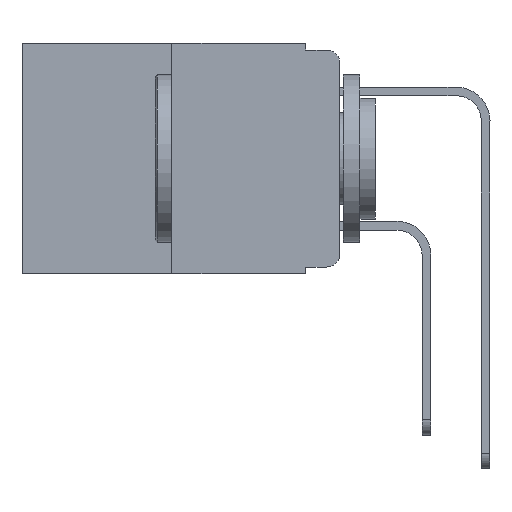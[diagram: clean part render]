
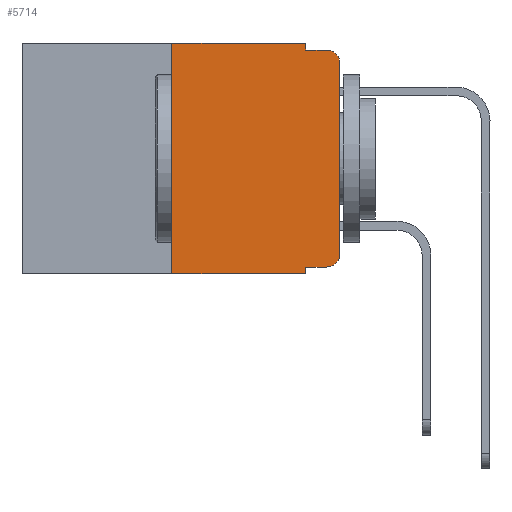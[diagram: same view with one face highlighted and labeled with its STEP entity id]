
A CAD part, left-side view. The second image highlights one B-rep face of the part: STEP entity #5714.
In plain terms, the highlighted planar face has unit normal (-1, 0, 0).
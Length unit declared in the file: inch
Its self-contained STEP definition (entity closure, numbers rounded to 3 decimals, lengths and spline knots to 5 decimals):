
#131 = VERTEX_POINT ( 'NONE', #2396 ) ;
#671 = CARTESIAN_POINT ( 'NONE',  ( 0., 0.051, 0. ) ) ;
#783 = AXIS2_PLACEMENT_3D ( 'NONE', #6863, #4051, #10195 ) ;
#1000 = DIRECTION ( 'NONE',  ( 0., 0., -1. ) ) ;
#1332 = LINE ( 'NONE', #9382, #6389 ) ;
#1361 = LINE ( 'NONE', #9855, #4149 ) ;
#1840 = CARTESIAN_POINT ( 'NONE',  ( 0., 0.25, 0. ) ) ;
#2251 = VERTEX_POINT ( 'NONE', #11145 ) ;
#2294 = DIRECTION ( 'NONE',  ( 0., -1., 0. ) ) ;
#2305 = EDGE_CURVE ( 'NONE', #131, #3315, #7604, .T. ) ;
#2396 = CARTESIAN_POINT ( 'NONE',  ( 0., 0.25, 0. ) ) ;
#2645 = CARTESIAN_POINT ( 'NONE',  ( 0., 0.051, 0. ) ) ;
#2754 = VECTOR ( 'NONE', #7580, 39.37008 ) ;
#2780 = ORIENTED_EDGE ( 'NONE', *, *, #8058, .T. ) ;
#2815 = ORIENTED_EDGE ( 'NONE', *, *, #8389, .T. ) ;
#2819 = EDGE_CURVE ( 'NONE', #5013, #5058, #1361, .T. ) ;
#2856 = ORIENTED_EDGE ( 'NONE', *, *, #8532, .F. ) ;
#2894 = ORIENTED_EDGE ( 'NONE', *, *, #8659, .F. ) ;
#2931 = ORIENTED_EDGE ( 'NONE', *, *, #2305, .F. ) ;
#3083 = PLANE ( 'NONE',  #783 ) ;
#3235 = ORIENTED_EDGE ( 'NONE', *, *, #8673, .F. ) ;
#3315 = VERTEX_POINT ( 'NONE', #2645 ) ;
#3355 = VERTEX_POINT ( 'NONE', #4920 ) ;
#3443 = ORIENTED_EDGE ( 'NONE', *, *, #2819, .T. ) ;
#3544 = VECTOR ( 'NONE', #9091, 39.37008 ) ;
#3650 = CARTESIAN_POINT ( 'NONE',  ( 0., 0., 0. ) ) ;
#3696 = ORIENTED_EDGE ( 'NONE', *, *, #8714, .F. ) ;
#3763 = ORIENTED_EDGE ( 'NONE', *, *, #8881, .T. ) ;
#4034 = ORIENTED_EDGE ( 'NONE', *, *, #8945, .T. ) ;
#4051 = DIRECTION ( 'NONE',  ( 1., 0., 0. ) ) ;
#4149 = VECTOR ( 'NONE', #9217, 39.37008 ) ;
#4359 = FACE_OUTER_BOUND ( 'NONE', #4909, .T. ) ;
#4392 = CARTESIAN_POINT ( 'NONE',  ( 0., 0.051, -0.01 ) ) ;
#4402 = DIRECTION ( 'NONE',  ( -1., 0., 0. ) ) ;
#4891 = LINE ( 'NONE', #8828, #7055 ) ;
#4909 = EDGE_LOOP ( 'NONE', ( #2780, #2815, #2856, #2894, #2931, #3235, #3443, #3696, #3763, #4034 ) ) ;
#4920 = CARTESIAN_POINT ( 'NONE',  ( 0., 0., -0.03 ) ) ;
#5013 = VERTEX_POINT ( 'NONE', #10700 ) ;
#5058 = VERTEX_POINT ( 'NONE', #11547 ) ;
#5257 = VECTOR ( 'NONE', #9611, 39.37008 ) ;
#5596 = DIRECTION ( 'NONE',  ( 0., -1., 0. ) ) ;
#5714 = ADVANCED_FACE ( 'NONE', ( #4359 ), #3083, .F. ) ;
#5864 = VERTEX_POINT ( 'NONE', #11930 ) ;
#5903 = VERTEX_POINT ( 'NONE', #4392 ) ;
#6389 = VECTOR ( 'NONE', #8623, 39.37008 ) ;
#6764 = DIRECTION ( 'NONE',  ( 0., 0., 1. ) ) ;
#6863 = CARTESIAN_POINT ( 'NONE',  ( 0., 0.473, 0. ) ) ;
#6985 = DIRECTION ( 'NONE',  ( -1., 0., 0. ) ) ;
#7055 = VECTOR ( 'NONE', #2294, 39.37008 ) ;
#7300 = VECTOR ( 'NONE', #5596, 39.37008 ) ;
#7331 = CARTESIAN_POINT ( 'NONE',  ( 0., 0.02, -0.01 ) ) ;
#7580 = DIRECTION ( 'NONE',  ( 0., 0., -1. ) ) ;
#7604 = LINE ( 'NONE', #8276, #5257 ) ;
#8058 = EDGE_CURVE ( 'NONE', #5864, #3355, #8150, .T. ) ;
#8150 = LINE ( 'NONE', #3650, #3544 ) ;
#8276 = CARTESIAN_POINT ( 'NONE',  ( 0., 0.473, 0. ) ) ;
#8389 = EDGE_CURVE ( 'NONE', #3355, #11373, #9450, .T. ) ;
#8532 = EDGE_CURVE ( 'NONE', #5903, #11373, #9570, .T. ) ;
#8623 = DIRECTION ( 'NONE',  ( 0., 0., -1. ) ) ;
#8659 = EDGE_CURVE ( 'NONE', #3315, #5903, #9929, .T. ) ;
#8673 = EDGE_CURVE ( 'NONE', #5013, #131, #11972, .T. ) ;
#8714 = EDGE_CURVE ( 'NONE', #2251, #5058, #1332, .T. ) ;
#8821 = CIRCLE ( 'NONE', #11505, 0.02 ) ;
#8828 = CARTESIAN_POINT ( 'NONE',  ( 0., 0.051, -0.333 ) ) ;
#8852 = CARTESIAN_POINT ( 'NONE',  ( 0., 0.02, -0.333 ) ) ;
#8881 = EDGE_CURVE ( 'NONE', #2251, #11107, #4891, .T. ) ;
#8945 = EDGE_CURVE ( 'NONE', #11107, #5864, #8821, .T. ) ;
#9079 = CARTESIAN_POINT ( 'NONE',  ( 0., 0.051, -0.01 ) ) ;
#9091 = DIRECTION ( 'NONE',  ( 0., 0., 1. ) ) ;
#9217 = DIRECTION ( 'NONE',  ( 0., -1., 0. ) ) ;
#9382 = CARTESIAN_POINT ( 'NONE',  ( 0., 0.051, 0. ) ) ;
#9450 = CIRCLE ( 'NONE', #9830, 0.02 ) ;
#9570 = LINE ( 'NONE', #9079, #7300 ) ;
#9611 = DIRECTION ( 'NONE',  ( 0., -1., 0. ) ) ;
#9682 = CARTESIAN_POINT ( 'NONE',  ( 0., 0.02, -0.313 ) ) ;
#9683 = VECTOR ( 'NONE', #6764, 39.37008 ) ;
#9830 = AXIS2_PLACEMENT_3D ( 'NONE', #11818, #6985, #1000 ) ;
#9855 = CARTESIAN_POINT ( 'NONE',  ( 0., 0.473, -0.343 ) ) ;
#9929 = LINE ( 'NONE', #671, #2754 ) ;
#10195 = DIRECTION ( 'NONE',  ( 0., 0., -1. ) ) ;
#10491 = DIRECTION ( 'NONE',  ( 0., 0., -1. ) ) ;
#10700 = CARTESIAN_POINT ( 'NONE',  ( 0., 0.25, -0.343 ) ) ;
#11107 = VERTEX_POINT ( 'NONE', #8852 ) ;
#11145 = CARTESIAN_POINT ( 'NONE',  ( 0., 0.051, -0.333 ) ) ;
#11373 = VERTEX_POINT ( 'NONE', #7331 ) ;
#11505 = AXIS2_PLACEMENT_3D ( 'NONE', #9682, #4402, #10491 ) ;
#11547 = CARTESIAN_POINT ( 'NONE',  ( 0., 0.051, -0.343 ) ) ;
#11818 = CARTESIAN_POINT ( 'NONE',  ( 0., 0.02, -0.03 ) ) ;
#11930 = CARTESIAN_POINT ( 'NONE',  ( 0., 0., -0.313 ) ) ;
#11972 = LINE ( 'NONE', #1840, #9683 ) ;
